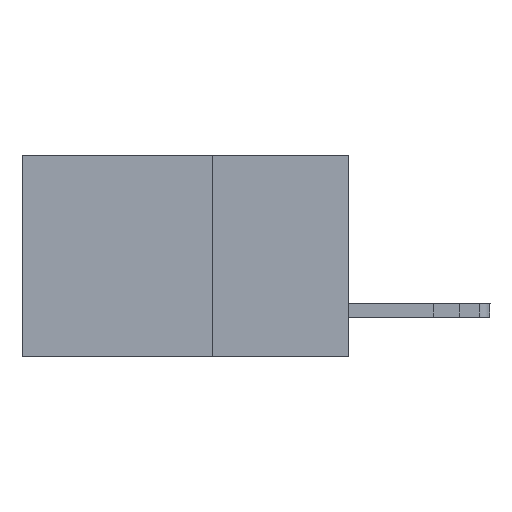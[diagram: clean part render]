
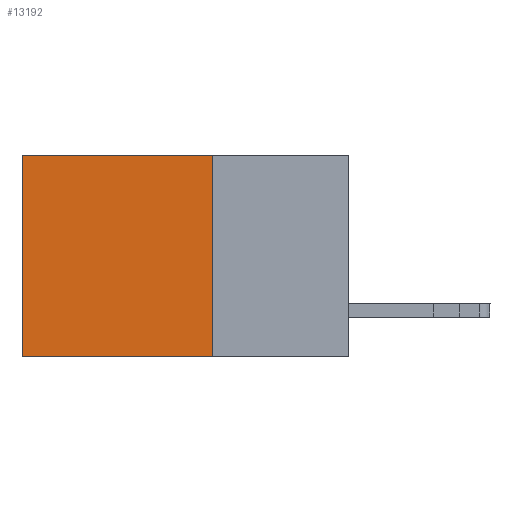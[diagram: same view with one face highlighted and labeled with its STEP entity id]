
A CAD part, left-side view. The second image highlights one B-rep face of the part: STEP entity #13192.
In plain terms, the highlighted planar face has unit normal (-1, 0, 0).
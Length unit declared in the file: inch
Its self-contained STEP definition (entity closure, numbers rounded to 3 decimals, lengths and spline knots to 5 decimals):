
#43 = ORIENTED_EDGE ( 'NONE', *, *, #2762, .F. ) ;
#127 = VECTOR ( 'NONE', #1986, 39.37008 ) ;
#300 = VERTEX_POINT ( 'NONE', #14430 ) ;
#1164 = VERTEX_POINT ( 'NONE', #15028 ) ;
#1785 = VERTEX_POINT ( 'NONE', #15483 ) ;
#1986 = DIRECTION ( 'NONE',  ( 0., 0., -1. ) ) ;
#2762 = EDGE_CURVE ( 'NONE', #300, #10080, #9442, .T. ) ;
#3775 = ORIENTED_EDGE ( 'NONE', *, *, #4941, .T. ) ;
#4139 = FACE_OUTER_BOUND ( 'NONE', #13889, .T. ) ;
#4442 = CARTESIAN_POINT ( 'NONE',  ( 0.2615, 0.6, -0.37 ) ) ;
#4941 = EDGE_CURVE ( 'NONE', #1164, #10080, #6639, .T. ) ;
#5062 = DIRECTION ( 'NONE',  ( 0., 0., -1. ) ) ;
#5130 = CARTESIAN_POINT ( 'NONE',  ( 0.2615, 0.25, 0. ) ) ;
#5212 = CARTESIAN_POINT ( 'NONE',  ( 0.2615, 0.6, -0.37 ) ) ;
#5266 = EDGE_CURVE ( 'NONE', #1785, #1164, #14146, .T. ) ;
#5966 = CARTESIAN_POINT ( 'NONE',  ( 0.2615, 0.25, -0.37 ) ) ;
#6018 = DIRECTION ( 'NONE',  ( 0., 1., 0. ) ) ;
#6189 = VECTOR ( 'NONE', #6018, 39.37008 ) ;
#6639 = LINE ( 'NONE', #4442, #127 ) ;
#7730 = ORIENTED_EDGE ( 'NONE', *, *, #9518, .F. ) ;
#8312 = AXIS2_PLACEMENT_3D ( 'NONE', #9839, #12300, #5062 ) ;
#9442 = LINE ( 'NONE', #5966, #6189 ) ;
#9518 = EDGE_CURVE ( 'NONE', #1785, #300, #13644, .T. ) ;
#9839 = CARTESIAN_POINT ( 'NONE',  ( 0.2615, 0.25, -0.37 ) ) ;
#10080 = VERTEX_POINT ( 'NONE', #5212 ) ;
#10137 = VECTOR ( 'NONE', #14966, 39.37008 ) ;
#11379 = VECTOR ( 'NONE', #13534, 39.37008 ) ;
#12300 = DIRECTION ( 'NONE',  ( 1., 0., 0. ) ) ;
#13192 = ADVANCED_FACE ( 'NONE', ( #4139 ), #14634, .F. ) ;
#13534 = DIRECTION ( 'NONE',  ( 0., 1., 0. ) ) ;
#13599 = ORIENTED_EDGE ( 'NONE', *, *, #5266, .T. ) ;
#13644 = LINE ( 'NONE', #13731, #10137 ) ;
#13731 = CARTESIAN_POINT ( 'NONE',  ( 0.2615, 0.25, -0.37 ) ) ;
#13889 = EDGE_LOOP ( 'NONE', ( #3775, #43, #7730, #13599 ) ) ;
#14146 = LINE ( 'NONE', #5130, #11379 ) ;
#14430 = CARTESIAN_POINT ( 'NONE',  ( 0.2615, 0.25, -0.37 ) ) ;
#14634 = PLANE ( 'NONE',  #8312 ) ;
#14966 = DIRECTION ( 'NONE',  ( 0., 0., -1. ) ) ;
#15028 = CARTESIAN_POINT ( 'NONE',  ( 0.2615, 0.6, 0. ) ) ;
#15483 = CARTESIAN_POINT ( 'NONE',  ( 0.2615, 0.25, 0. ) ) ;
